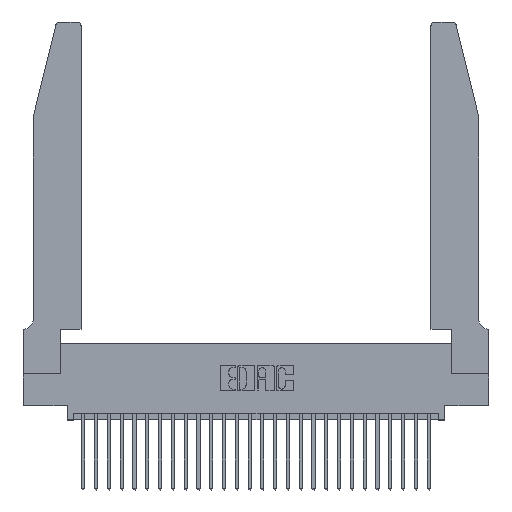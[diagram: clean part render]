
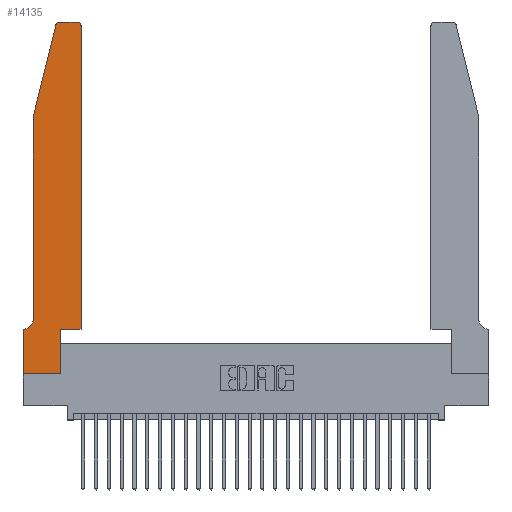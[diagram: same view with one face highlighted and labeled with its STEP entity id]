
A CAD part, top view. The second image highlights one B-rep face of the part: STEP entity #14135.
In plain terms, the highlighted planar face has unit normal (0, 0, 1).
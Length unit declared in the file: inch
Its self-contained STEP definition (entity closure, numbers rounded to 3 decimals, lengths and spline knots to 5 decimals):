
#187 = ORIENTED_EDGE ( 'NONE', *, *, #3895, .T. ) ;
#206 = CARTESIAN_POINT ( 'NONE',  ( 0.0755, 2., 0.37 ) ) ;
#566 = VERTEX_POINT ( 'NONE', #3182 ) ;
#769 = CARTESIAN_POINT ( 'NONE',  ( 0.2865, 0., 0.37 ) ) ;
#1245 = CIRCLE ( 'NONE', #16504, 0.03 ) ;
#1582 = CIRCLE ( 'NONE', #24604, 0.03 ) ;
#1679 = EDGE_CURVE ( 'NONE', #2929, #19790, #28751, .T. ) ;
#1921 = VERTEX_POINT ( 'NONE', #769 ) ;
#2215 = LINE ( 'NONE', #20443, #19559 ) ;
#2400 = VERTEX_POINT ( 'NONE', #11524 ) ;
#2631 = CARTESIAN_POINT ( 'NONE',  ( 0.4505, 0.35, 0.37 ) ) ;
#2635 = EDGE_CURVE ( 'NONE', #19790, #1921, #15836, .T. ) ;
#2822 = DIRECTION ( 'NONE',  ( 1., 0., 0. ) ) ;
#2929 = VERTEX_POINT ( 'NONE', #19739 ) ;
#2942 = VERTEX_POINT ( 'NONE', #6944 ) ;
#3182 = CARTESIAN_POINT ( 'NONE',  ( 0.4505, 2.72, 0.37 ) ) ;
#3193 = EDGE_CURVE ( 'NONE', #566, #2942, #1582, .T. ) ;
#3205 = CARTESIAN_POINT ( 'NONE',  ( 0.25487, 2.72718, 0.37 ) ) ;
#3459 = ORIENTED_EDGE ( 'NONE', *, *, #23672, .T. ) ;
#3895 = EDGE_CURVE ( 'NONE', #2400, #6681, #16851, .T. ) ;
#3932 = ORIENTED_EDGE ( 'NONE', *, *, #24412, .T. ) ;
#4429 = CARTESIAN_POINT ( 'NONE',  ( 0.4505, 0.35, 0.37 ) ) ;
#4623 = ORIENTED_EDGE ( 'NONE', *, *, #23083, .T. ) ;
#5039 = DIRECTION ( 'NONE',  ( -0.239, -0.971, 0. ) ) ;
#5092 = DIRECTION ( 'NONE',  ( -1., 0., 0. ) ) ;
#5110 = DIRECTION ( 'NONE',  ( 0., 1., 0. ) ) ;
#5239 = LINE ( 'NONE', #16584, #13226 ) ;
#5418 = VERTEX_POINT ( 'NONE', #13045 ) ;
#5651 = AXIS2_PLACEMENT_3D ( 'NONE', #12800, #28213, #28131 ) ;
#5861 = LINE ( 'NONE', #13891, #28768 ) ;
#6407 = ORIENTED_EDGE ( 'NONE', *, *, #21219, .T. ) ;
#6681 = VERTEX_POINT ( 'NONE', #4429 ) ;
#6869 = ORIENTED_EDGE ( 'NONE', *, *, #26391, .T. ) ;
#6910 = ORIENTED_EDGE ( 'NONE', *, *, #7186, .T. ) ;
#6944 = CARTESIAN_POINT ( 'NONE',  ( 0.4205, 2.75, 0.37 ) ) ;
#7123 = VECTOR ( 'NONE', #5039, 39.37008 ) ;
#7186 = EDGE_CURVE ( 'NONE', #19118, #2929, #15699, .T. ) ;
#7254 = DIRECTION ( 'NONE',  ( 0., -1., 0. ) ) ;
#7325 = CARTESIAN_POINT ( 'NONE',  ( 0.0755, 0.35, 0.37 ) ) ;
#7747 = ORIENTED_EDGE ( 'NONE', *, *, #2635, .T. ) ;
#7935 = VECTOR ( 'NONE', #26903, 39.37008 ) ;
#8798 = VERTEX_POINT ( 'NONE', #206 ) ;
#9075 = CARTESIAN_POINT ( 'NONE',  ( 0.284, 2.72, 0.37 ) ) ;
#9499 = VERTEX_POINT ( 'NONE', #20761 ) ;
#9534 = DIRECTION ( 'NONE',  ( -1., 0., 0. ) ) ;
#9796 = VECTOR ( 'NONE', #9534, 39.37008 ) ;
#10290 = AXIS2_PLACEMENT_3D ( 'NONE', #12527, #12615, #16976 ) ;
#10990 = CARTESIAN_POINT ( 'NONE',  ( 0., 0., 0.37 ) ) ;
#11524 = CARTESIAN_POINT ( 'NONE',  ( 0.2865, 0.35, 0.37 ) ) ;
#12024 = VECTOR ( 'NONE', #2822, 39.37008 ) ;
#12527 = CARTESIAN_POINT ( 'NONE',  ( 0.0055, 0.42, 0.37 ) ) ;
#12615 = DIRECTION ( 'NONE',  ( 0., 0., -1. ) ) ;
#12800 = CARTESIAN_POINT ( 'NONE',  ( 0., 0.35, 0.37 ) ) ;
#12923 = VECTOR ( 'NONE', #7254, 39.37008 ) ;
#13045 = CARTESIAN_POINT ( 'NONE',  ( 0.0755, 0.42, 0.37 ) ) ;
#13226 = VECTOR ( 'NONE', #23290, 39.37008 ) ;
#13328 = CARTESIAN_POINT ( 'NONE',  ( 0., 0., 0.37 ) ) ;
#13830 = CARTESIAN_POINT ( 'NONE',  ( 0.0055, 0.35, 0.37 ) ) ;
#13891 = CARTESIAN_POINT ( 'NONE',  ( 0.2605, 2.75, 0.37 ) ) ;
#13930 = CARTESIAN_POINT ( 'NONE',  ( 0.0755, 2., 0.37 ) ) ;
#14135 = ADVANCED_FACE ( 'NONE', ( #26164 ), #23491, .T. ) ;
#14191 = EDGE_LOOP ( 'NONE', ( #17139, #6407, #4623, #6869, #3932, #6910, #15567, #7747, #3459, #187, #28621, #14204 ) ) ;
#14204 = ORIENTED_EDGE ( 'NONE', *, *, #3193, .T. ) ;
#15529 = DIRECTION ( 'NONE',  ( 1., 0., 0. ) ) ;
#15567 = ORIENTED_EDGE ( 'NONE', *, *, #1679, .T. ) ;
#15699 = LINE ( 'NONE', #7325, #9796 ) ;
#15748 = VERTEX_POINT ( 'NONE', #3205 ) ;
#15836 = LINE ( 'NONE', #10990, #16540 ) ;
#15855 = CARTESIAN_POINT ( 'NONE',  ( 0.0755, 2., 0.37 ) ) ;
#15859 = EDGE_CURVE ( 'NONE', #6681, #566, #5239, .T. ) ;
#16504 = AXIS2_PLACEMENT_3D ( 'NONE', #9075, #26819, #28777 ) ;
#16540 = VECTOR ( 'NONE', #15529, 39.37008 ) ;
#16584 = CARTESIAN_POINT ( 'NONE',  ( 0.4505, 0.35, 0.37 ) ) ;
#16851 = LINE ( 'NONE', #2631, #12024 ) ;
#16976 = DIRECTION ( 'NONE',  ( -1., 0., 0. ) ) ;
#17114 = DIRECTION ( 'NONE',  ( 1., 0., 0. ) ) ;
#17139 = ORIENTED_EDGE ( 'NONE', *, *, #17154, .T. ) ;
#17154 = EDGE_CURVE ( 'NONE', #2942, #9499, #5861, .T. ) ;
#17438 = LINE ( 'NONE', #15855, #12923 ) ;
#18463 = CARTESIAN_POINT ( 'NONE',  ( 0., 0., 0.37 ) ) ;
#19118 = VERTEX_POINT ( 'NONE', #13830 ) ;
#19559 = VECTOR ( 'NONE', #5110, 39.37008 ) ;
#19739 = CARTESIAN_POINT ( 'NONE',  ( 0., 0.35, 0.37 ) ) ;
#19790 = VERTEX_POINT ( 'NONE', #18463 ) ;
#20443 = CARTESIAN_POINT ( 'NONE',  ( 0.2865, 0.35, 0.37 ) ) ;
#20761 = CARTESIAN_POINT ( 'NONE',  ( 0.284, 2.75, 0.37 ) ) ;
#21219 = EDGE_CURVE ( 'NONE', #9499, #15748, #1245, .T. ) ;
#22727 = LINE ( 'NONE', #13930, #7123 ) ;
#23083 = EDGE_CURVE ( 'NONE', #15748, #8798, #22727, .T. ) ;
#23290 = DIRECTION ( 'NONE',  ( 0., 1., 0. ) ) ;
#23491 = PLANE ( 'NONE',  #5651 ) ;
#23640 = DIRECTION ( 'NONE',  ( 0., 0., 1. ) ) ;
#23672 = EDGE_CURVE ( 'NONE', #1921, #2400, #2215, .T. ) ;
#24412 = EDGE_CURVE ( 'NONE', #5418, #19118, #26133, .T. ) ;
#24604 = AXIS2_PLACEMENT_3D ( 'NONE', #25850, #23640, #17114 ) ;
#25850 = CARTESIAN_POINT ( 'NONE',  ( 0.4205, 2.72, 0.37 ) ) ;
#26133 = CIRCLE ( 'NONE', #10290, 0.07 ) ;
#26164 = FACE_OUTER_BOUND ( 'NONE', #14191, .T. ) ;
#26391 = EDGE_CURVE ( 'NONE', #8798, #5418, #17438, .T. ) ;
#26819 = DIRECTION ( 'NONE',  ( 0., 0., 1. ) ) ;
#26903 = DIRECTION ( 'NONE',  ( 0., -1., 0. ) ) ;
#28131 = DIRECTION ( 'NONE',  ( 1., 0., 0. ) ) ;
#28213 = DIRECTION ( 'NONE',  ( 0., 0., 1. ) ) ;
#28621 = ORIENTED_EDGE ( 'NONE', *, *, #15859, .T. ) ;
#28751 = LINE ( 'NONE', #13328, #7935 ) ;
#28768 = VECTOR ( 'NONE', #5092, 39.37008 ) ;
#28777 = DIRECTION ( 'NONE',  ( 1., 0., 0. ) ) ;
